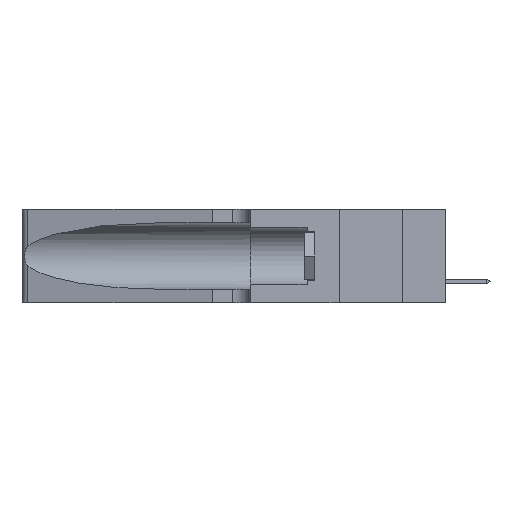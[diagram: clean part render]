
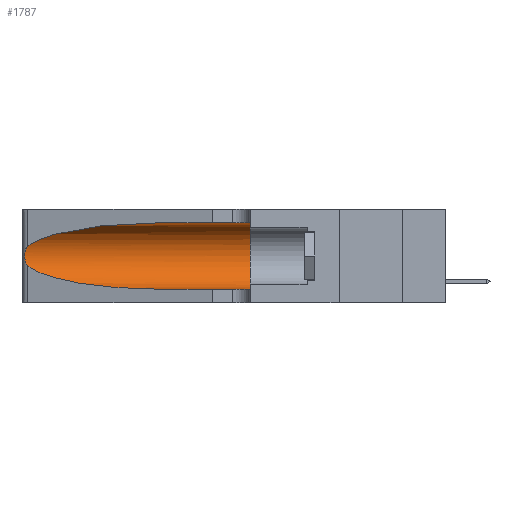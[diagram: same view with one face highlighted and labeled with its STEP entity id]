
A CAD part, left-side view. The second image highlights one B-rep face of the part: STEP entity #1787.
In plain terms, the highlighted cylindrical face has radius 3.308 mm (diameter 6.617 mm), a partial arc.
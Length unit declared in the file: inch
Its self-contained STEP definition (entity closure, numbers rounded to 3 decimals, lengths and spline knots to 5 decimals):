
#361 = CARTESIAN_POINT ( 'NONE',  ( 0.26017, 1.23833, 0.17102 ) ) ;
#857 = EDGE_LOOP ( 'NONE', ( #4560, #6108, #8195, #15442, #4366, #14403 ) ) ;
#1200 = EDGE_CURVE ( 'NONE', #9217, #6446, #15323, .T. ) ;
#1539 = CARTESIAN_POINT ( 'NONE',  ( 0.25787, 1.23484, 0.2124 ) ) ;
#1606 = CARTESIAN_POINT ( 'NONE',  ( 0.26018, 1.23835, 0.19895 ) ) ;
#1787 = ADVANCED_FACE ( 'NONE', ( #19071 ), #16250, .F. ) ;
#2193 = CARTESIAN_POINT ( 'NONE',  ( 0.25555, 1.22993, 0.14849 ) ) ;
#2712 = AXIS2_PLACEMENT_3D ( 'NONE', #16823, #20778, #18683 ) ;
#3116 = EDGE_CURVE ( 'NONE', #9217, #14270, #11065, .T. ) ;
#3903 = VERTEX_POINT ( 'NONE', #14187 ) ;
#4366 = ORIENTED_EDGE ( 'NONE', *, *, #7922, .F. ) ;
#4529 = EDGE_CURVE ( 'NONE', #10092, #3903, #7767, .T. ) ;
#4560 = ORIENTED_EDGE ( 'NONE', *, *, #1200, .T. ) ;
#4664 = CARTESIAN_POINT ( 'NONE',  ( 0.25487, 1.22718, 0.22369 ) ) ;
#4678 = B_SPLINE_CURVE_WITH_KNOTS ( 'NONE', 3,
 ( #4664, #16081, #19394, #1539, #19459, #1606, #16587, #12417, #361, #14838, #6575, #8509, #2193, #15189 ),
 .UNSPECIFIED., .F., .F.,
 ( 4, 2, 2, 2, 2, 2, 4 ),
 ( 0., 0.00027, 0.00053, 0.00107, 0.0016, 0.00187, 0.00214 ),
 .UNSPECIFIED. ) ;
#5270 = EDGE_CURVE ( 'NONE', #6446, #10092, #4678, .T. ) ;
#5484 = CARTESIAN_POINT ( 'NONE',  ( 0.1305, 0.35, 0.31525 ) ) ;
#6108 = ORIENTED_EDGE ( 'NONE', *, *, #5270, .T. ) ;
#6446 = VERTEX_POINT ( 'NONE', #18908 ) ;
#6575 = CARTESIAN_POINT ( 'NONE',  ( 0.25789, 1.23486, 0.15765 ) ) ;
#6839 = CARTESIAN_POINT ( 'NONE',  ( 0.1305, 0.35, 0.185 ) ) ;
#7548 = CARTESIAN_POINT ( 'NONE',  ( 0.25487, 1.22718, 0.14631 ) ) ;
#7612 = CARTESIAN_POINT ( 'NONE',  ( 0.18966, 0.96281, 0.05475 ) ) ;
#7767 =( BOUNDED_CURVE ( )  B_SPLINE_CURVE ( 3, ( #7548, #8978, #7612, #10785 ),
 .UNSPECIFIED., .F., .T. ) 
 B_SPLINE_CURVE_WITH_KNOTS ( ( 4, 4 ),
 ( 3.44316, 4.71239 ),
 .UNSPECIFIED. ) 
 CURVE ( )  GEOMETRIC_REPRESENTATION_ITEM ( )  RATIONAL_B_SPLINE_CURVE ( ( 1., 0.87, 0.87, 1. ) ) 
 REPRESENTATION_ITEM ( '' )  );
#7833 = CARTESIAN_POINT ( 'NONE',  ( 0.1305, 0.72297, 0.31525 ) ) ;
#7922 = EDGE_CURVE ( 'NONE', #14270, #19615, #9740, .T. ) ;
#8195 = ORIENTED_EDGE ( 'NONE', *, *, #4529, .T. ) ;
#8386 = VECTOR ( 'NONE', #11445, 39.37008 ) ;
#8509 = CARTESIAN_POINT ( 'NONE',  ( 0.25639, 1.23186, 0.15144 ) ) ;
#8978 = CARTESIAN_POINT ( 'NONE',  ( 0.2373, 1.15595, 0.08982 ) ) ;
#9217 = VERTEX_POINT ( 'NONE', #11253 ) ;
#9740 = CIRCLE ( 'NONE', #19848, 0.13025 ) ;
#10054 = VECTOR ( 'NONE', #17226, 39.37008 ) ;
#10092 = VERTEX_POINT ( 'NONE', #10677 ) ;
#10677 = CARTESIAN_POINT ( 'NONE',  ( 0.25487, 1.22718, 0.14631 ) ) ;
#10785 = CARTESIAN_POINT ( 'NONE',  ( 0.1305, 0.72297, 0.05475 ) ) ;
#10989 = CARTESIAN_POINT ( 'NONE',  ( 0.25487, 1.22718, 0.22369 ) ) ;
#11065 = LINE ( 'NONE', #15568, #10054 ) ;
#11253 = CARTESIAN_POINT ( 'NONE',  ( 0.1305, 0.72297, 0.31525 ) ) ;
#11290 = CARTESIAN_POINT ( 'NONE',  ( 0.1305, 0.35, 0.05475 ) ) ;
#11445 = DIRECTION ( 'NONE',  ( 0., -1., 0. ) ) ;
#12417 = CARTESIAN_POINT ( 'NONE',  ( 0.26075, 1.23896, 0.178 ) ) ;
#12700 = LINE ( 'NONE', #16385, #8386 ) ;
#14187 = CARTESIAN_POINT ( 'NONE',  ( 0.1305, 0.72297, 0.05475 ) ) ;
#14270 = VERTEX_POINT ( 'NONE', #5484 ) ;
#14403 = ORIENTED_EDGE ( 'NONE', *, *, #3116, .F. ) ;
#14838 = CARTESIAN_POINT ( 'NONE',  ( 0.25856, 1.23593, 0.16098 ) ) ;
#15189 = CARTESIAN_POINT ( 'NONE',  ( 0.25487, 1.22718, 0.14631 ) ) ;
#15323 =( BOUNDED_CURVE ( )  B_SPLINE_CURVE ( 3, ( #7833, #20872, #15863, #10989 ),
 .UNSPECIFIED., .F., .F. ) 
 B_SPLINE_CURVE_WITH_KNOTS ( ( 4, 4 ),
 ( 1.5708, 2.84003 ),
 .UNSPECIFIED. ) 
 CURVE ( )  GEOMETRIC_REPRESENTATION_ITEM ( )  RATIONAL_B_SPLINE_CURVE ( ( 1., 0.87, 0.87, 1. ) ) 
 REPRESENTATION_ITEM ( '' )  );
#15442 = ORIENTED_EDGE ( 'NONE', *, *, #19212, .T. ) ;
#15568 = CARTESIAN_POINT ( 'NONE',  ( 0.1305, 1.61858, 0.31525 ) ) ;
#15863 = CARTESIAN_POINT ( 'NONE',  ( 0.2373, 1.15595, 0.28018 ) ) ;
#15903 = DIRECTION ( 'NONE',  ( 0., 0., 1. ) ) ;
#16081 = CARTESIAN_POINT ( 'NONE',  ( 0.25555, 1.22994, 0.2215 ) ) ;
#16250 = CYLINDRICAL_SURFACE ( 'NONE', #2712, 0.13025 ) ;
#16385 = CARTESIAN_POINT ( 'NONE',  ( 0.1305, 1.61858, 0.05475 ) ) ;
#16587 = CARTESIAN_POINT ( 'NONE',  ( 0.26075, 1.23896, 0.19203 ) ) ;
#16823 = CARTESIAN_POINT ( 'NONE',  ( 0.1305, 1.61858, 0.185 ) ) ;
#17226 = DIRECTION ( 'NONE',  ( 0., -1., 0. ) ) ;
#18474 = DIRECTION ( 'NONE',  ( 0., 1., 0. ) ) ;
#18683 = DIRECTION ( 'NONE',  ( 0., 0., -1. ) ) ;
#18908 = CARTESIAN_POINT ( 'NONE',  ( 0.25487, 1.22718, 0.22369 ) ) ;
#19071 = FACE_OUTER_BOUND ( 'NONE', #857, .T. ) ;
#19212 = EDGE_CURVE ( 'NONE', #3903, #19615, #12700, .T. ) ;
#19394 = CARTESIAN_POINT ( 'NONE',  ( 0.25639, 1.23184, 0.21858 ) ) ;
#19459 = CARTESIAN_POINT ( 'NONE',  ( 0.25854, 1.2359, 0.20912 ) ) ;
#19615 = VERTEX_POINT ( 'NONE', #11290 ) ;
#19848 = AXIS2_PLACEMENT_3D ( 'NONE', #6839, #18474, #15903 ) ;
#20778 = DIRECTION ( 'NONE',  ( 0., -1., 0. ) ) ;
#20872 = CARTESIAN_POINT ( 'NONE',  ( 0.18966, 0.96281, 0.31525 ) ) ;
